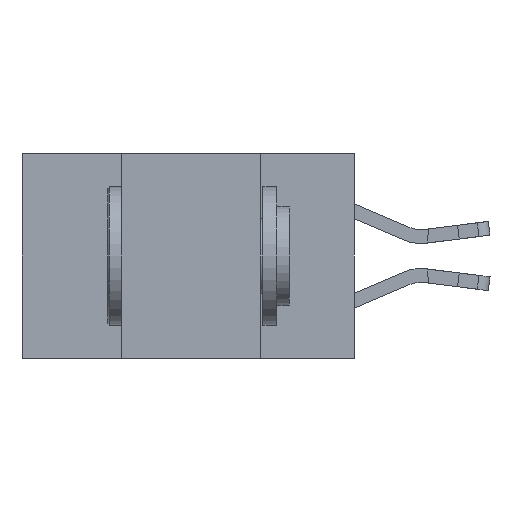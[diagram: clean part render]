
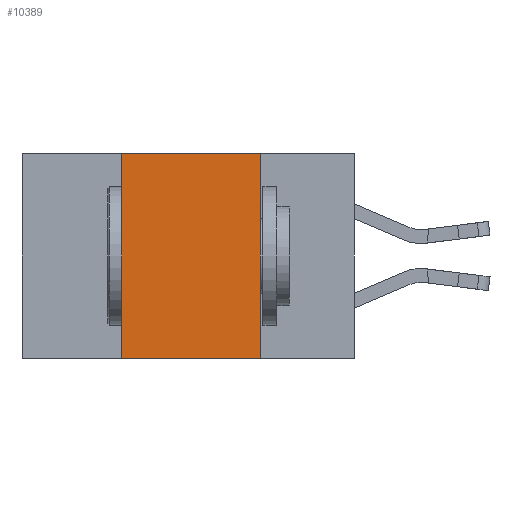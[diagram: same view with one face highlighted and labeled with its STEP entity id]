
A CAD part, left-side view. The second image highlights one B-rep face of the part: STEP entity #10389.
In plain terms, the highlighted planar face has unit normal (-1, 0, 0).
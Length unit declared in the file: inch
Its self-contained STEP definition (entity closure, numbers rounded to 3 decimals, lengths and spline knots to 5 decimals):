
#2 = EDGE_CURVE ( 'NONE', #25780, #18906, #2088, .T. ) ;
#1468 = EDGE_LOOP ( 'NONE', ( #16548, #27876, #7608, #16557 ) ) ;
#1921 = CARTESIAN_POINT ( 'NONE',  ( 0., 0.42, 0. ) ) ;
#2027 = VECTOR ( 'NONE', #11039, 39.37008 ) ;
#2088 = LINE ( 'NONE', #10916, #7594 ) ;
#2379 = LINE ( 'NONE', #19583, #2027 ) ;
#3968 = DIRECTION ( 'NONE',  ( 0., 0., -1. ) ) ;
#4380 = VERTEX_POINT ( 'NONE', #12705 ) ;
#7356 = CARTESIAN_POINT ( 'NONE',  ( 0., 0.6, -0.37 ) ) ;
#7594 = VECTOR ( 'NONE', #13122, 39.37008 ) ;
#7608 = ORIENTED_EDGE ( 'NONE', *, *, #2, .F. ) ;
#8424 = CARTESIAN_POINT ( 'NONE',  ( 0., 0.17, -0.37 ) ) ;
#8510 = CARTESIAN_POINT ( 'NONE',  ( 0., 0.6, 0. ) ) ;
#8577 = VERTEX_POINT ( 'NONE', #8424 ) ;
#9437 = DIRECTION ( 'NONE',  ( 0., -1., 0. ) ) ;
#10389 = ADVANCED_FACE ( 'NONE', ( #22978 ), #10414, .F. ) ;
#10414 = PLANE ( 'NONE',  #27315 ) ;
#10916 = CARTESIAN_POINT ( 'NONE',  ( 0., 0.42, 0. ) ) ;
#11039 = DIRECTION ( 'NONE',  ( 0., 0., -1. ) ) ;
#11467 = VECTOR ( 'NONE', #9437, 39.37008 ) ;
#11743 = CARTESIAN_POINT ( 'NONE',  ( 0., 0.6, 0. ) ) ;
#12705 = CARTESIAN_POINT ( 'NONE',  ( 0., 0.17, 0. ) ) ;
#13122 = DIRECTION ( 'NONE',  ( 0., 0., 1. ) ) ;
#16012 = EDGE_CURVE ( 'NONE', #18906, #4380, #27688, .T. ) ;
#16548 = ORIENTED_EDGE ( 'NONE', *, *, #27611, .F. ) ;
#16557 = ORIENTED_EDGE ( 'NONE', *, *, #19327, .T. ) ;
#16801 = LINE ( 'NONE', #7356, #24346 ) ;
#17960 = DIRECTION ( 'NONE',  ( 0., -1., 0. ) ) ;
#18906 = VERTEX_POINT ( 'NONE', #1921 ) ;
#19327 = EDGE_CURVE ( 'NONE', #25780, #8577, #16801, .T. ) ;
#19583 = CARTESIAN_POINT ( 'NONE',  ( 0., 0.17, 0. ) ) ;
#22978 = FACE_OUTER_BOUND ( 'NONE', #1468, .T. ) ;
#24346 = VECTOR ( 'NONE', #17960, 39.37008 ) ;
#25780 = VERTEX_POINT ( 'NONE', #26229 ) ;
#26229 = CARTESIAN_POINT ( 'NONE',  ( 0., 0.42, -0.37 ) ) ;
#27315 = AXIS2_PLACEMENT_3D ( 'NONE', #8510, #28251, #3968 ) ;
#27611 = EDGE_CURVE ( 'NONE', #4380, #8577, #2379, .T. ) ;
#27688 = LINE ( 'NONE', #11743, #11467 ) ;
#27876 = ORIENTED_EDGE ( 'NONE', *, *, #16012, .F. ) ;
#28251 = DIRECTION ( 'NONE',  ( 1., 0., 0. ) ) ;
